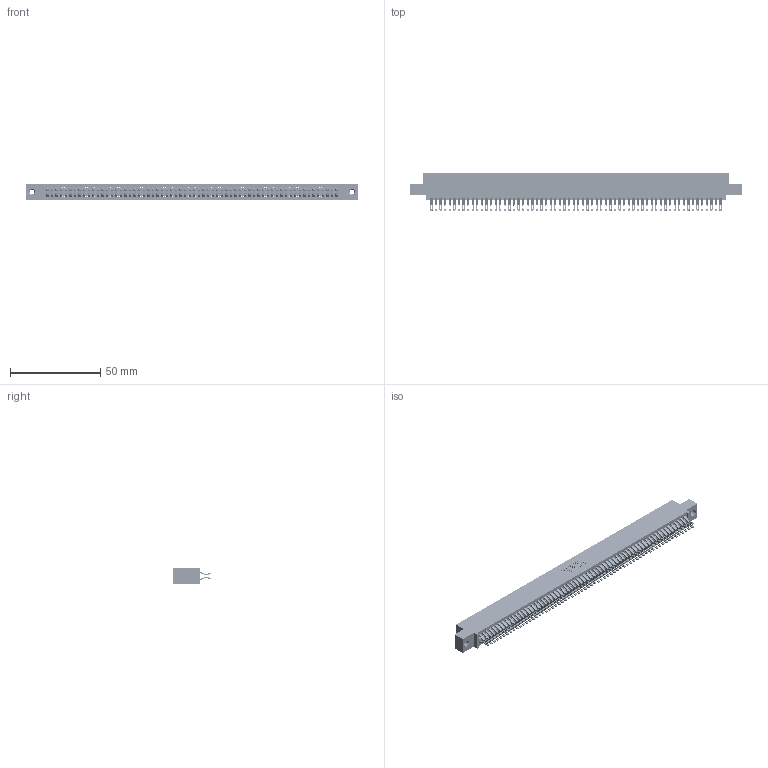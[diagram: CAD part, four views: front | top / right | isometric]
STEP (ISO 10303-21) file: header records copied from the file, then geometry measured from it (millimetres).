
FILE_DESCRIPTION (( 'STEP AP203' ), '1' );
FILE_NAME ('345-128-555-507.STEP', '2019-11-07T09:43:26', ( '' ), ( '' ), 'SwSTEP 2.0', 'SolidWorks 2016', '' );
FILE_SCHEMA (( 'CONFIG_CONTROL_DESIGN' ));
Length unit declared in the file: inch
Products named in the file (4): 345 Part_0.110 Offset - 0.156 Dia-TI; 345-128-555-507; 345-250-001_345-250-005-103; 345-292-001_555 Tail
Assembly tree (131 placements, depth 2):
  345-128-555-507
    345 Part_0.110 Offset - 0.156 Dia-TI
    345-292-001_555 Tail  x128
    345-250-001_345-250-005-103  x2
Bounding box: 183.77 x 21.13 x 9.4 mm (x, y, z)
Volume: 18340.1 mm3; surface area: 28947.9 mm2
Topology: 131 solids, 131 shells, 7358 faces, 23145 edges, 15422 vertices
Faces by surface type: plane 4084, cylinder 3258, cone 12, torus 4
Entity records: 48898 total; most frequent: CARTESIAN_POINT 8193, ORIENTED_EDGE 8090, DIRECTION 7191, EDGE_CURVE 4045, LINE 3617, VECTOR 3617, VERTEX_POINT 2692, AXIS2_PLACEMENT_3D 1787
